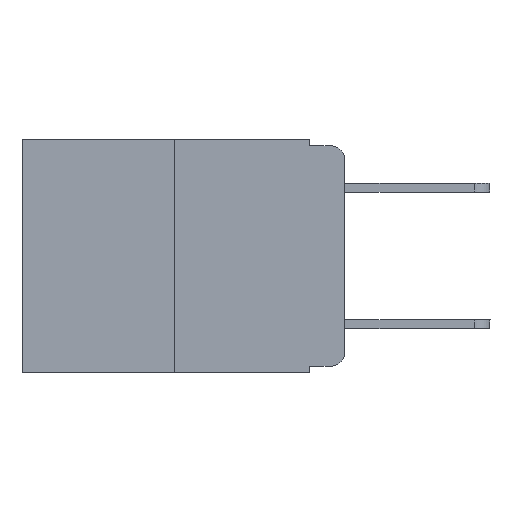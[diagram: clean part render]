
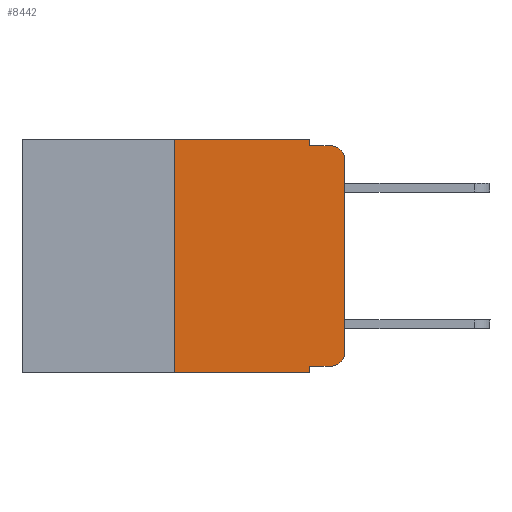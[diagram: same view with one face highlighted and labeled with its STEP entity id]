
A CAD part, left-side view. The second image highlights one B-rep face of the part: STEP entity #8442.
In plain terms, the highlighted planar face has unit normal (-1, 0, 0).
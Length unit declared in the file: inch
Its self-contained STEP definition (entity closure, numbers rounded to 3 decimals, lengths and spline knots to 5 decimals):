
#115 = LINE ( 'NONE', #10864, #8939 ) ;
#200 = LINE ( 'NONE', #6175, #12722 ) ;
#201 = EDGE_CURVE ( 'NONE', #2039, #1813, #435, .T. ) ;
#435 = LINE ( 'NONE', #6484, #12505 ) ;
#469 = ORIENTED_EDGE ( 'NONE', *, *, #7797, .T. ) ;
#483 = VECTOR ( 'NONE', #10882, 39.37008 ) ;
#596 = DIRECTION ( 'NONE',  ( 0., -1., 0. ) ) ;
#597 = CARTESIAN_POINT ( 'NONE',  ( 0., 0.051, -0.333 ) ) ;
#646 = DIRECTION ( 'NONE',  ( 0., -1., 0. ) ) ;
#672 = AXIS2_PLACEMENT_3D ( 'NONE', #8662, #4811, #8749 ) ;
#1133 = ORIENTED_EDGE ( 'NONE', *, *, #11712, .T. ) ;
#1342 = EDGE_LOOP ( 'NONE', ( #6219, #469, #8096, #11577, #10101, #4551, #4410, #12047, #10363, #1133 ) ) ;
#1742 = VECTOR ( 'NONE', #646, 39.37008 ) ;
#1813 = VERTEX_POINT ( 'NONE', #3310 ) ;
#1833 = CARTESIAN_POINT ( 'NONE',  ( 0., 0.25, -0.343 ) ) ;
#1901 = CARTESIAN_POINT ( 'NONE',  ( 0., 0.25, 0. ) ) ;
#1926 = VERTEX_POINT ( 'NONE', #1833 ) ;
#2039 = VERTEX_POINT ( 'NONE', #8715 ) ;
#2201 = VERTEX_POINT ( 'NONE', #11887 ) ;
#2207 = LINE ( 'NONE', #4011, #483 ) ;
#2269 = CARTESIAN_POINT ( 'NONE',  ( 0., 0., -0.03 ) ) ;
#2377 = CIRCLE ( 'NONE', #8976, 0.02 ) ;
#2406 = CARTESIAN_POINT ( 'NONE',  ( 0., 0., -0.313 ) ) ;
#2563 = LINE ( 'NONE', #6766, #8119 ) ;
#3084 = DIRECTION ( 'NONE',  ( 0., 0., 1. ) ) ;
#3139 = EDGE_CURVE ( 'NONE', #2201, #9923, #11011, .T. ) ;
#3310 = CARTESIAN_POINT ( 'NONE',  ( 0., 0.051, -0.01 ) ) ;
#3576 = VERTEX_POINT ( 'NONE', #2269 ) ;
#3888 = EDGE_CURVE ( 'NONE', #8419, #2039, #6986, .T. ) ;
#4011 = CARTESIAN_POINT ( 'NONE',  ( 0., 0.051, -0.01 ) ) ;
#4060 = LINE ( 'NONE', #8194, #5748 ) ;
#4410 = ORIENTED_EDGE ( 'NONE', *, *, #9126, .T. ) ;
#4491 = CIRCLE ( 'NONE', #672, 0.02 ) ;
#4504 = VERTEX_POINT ( 'NONE', #12550 ) ;
#4551 = ORIENTED_EDGE ( 'NONE', *, *, #7932, .F. ) ;
#4811 = DIRECTION ( 'NONE',  ( -1., 0., 0. ) ) ;
#5748 = VECTOR ( 'NONE', #9230, 39.37008 ) ;
#6021 = VERTEX_POINT ( 'NONE', #9377 ) ;
#6175 = CARTESIAN_POINT ( 'NONE',  ( 0., 0., 0. ) ) ;
#6219 = ORIENTED_EDGE ( 'NONE', *, *, #10910, .T. ) ;
#6456 = DIRECTION ( 'NONE',  ( -1., 0., 0. ) ) ;
#6484 = CARTESIAN_POINT ( 'NONE',  ( 0., 0.051, 0. ) ) ;
#6487 = CARTESIAN_POINT ( 'NONE',  ( 0., 0.02, -0.313 ) ) ;
#6766 = CARTESIAN_POINT ( 'NONE',  ( 0., 0.473, -0.343 ) ) ;
#6986 = LINE ( 'NONE', #10093, #1742 ) ;
#7739 = DIRECTION ( 'NONE',  ( 0., 0., -1. ) ) ;
#7797 = EDGE_CURVE ( 'NONE', #3576, #4504, #4491, .T. ) ;
#7932 = EDGE_CURVE ( 'NONE', #1926, #8419, #115, .T. ) ;
#8096 = ORIENTED_EDGE ( 'NONE', *, *, #11501, .F. ) ;
#8119 = VECTOR ( 'NONE', #596, 39.37008 ) ;
#8194 = CARTESIAN_POINT ( 'NONE',  ( 0., 0.051, 0. ) ) ;
#8419 = VERTEX_POINT ( 'NONE', #1901 ) ;
#8442 = ADVANCED_FACE ( 'NONE', ( #9376 ), #8820, .F. ) ;
#8536 = DIRECTION ( 'NONE',  ( 0., 0., -1. ) ) ;
#8662 = CARTESIAN_POINT ( 'NONE',  ( 0., 0.02, -0.03 ) ) ;
#8715 = CARTESIAN_POINT ( 'NONE',  ( 0., 0.051, 0. ) ) ;
#8739 = DIRECTION ( 'NONE',  ( 1., 0., 0. ) ) ;
#8749 = DIRECTION ( 'NONE',  ( 0., 0., -1. ) ) ;
#8820 = PLANE ( 'NONE',  #11857 ) ;
#8939 = VECTOR ( 'NONE', #3084, 39.37008 ) ;
#8976 = AXIS2_PLACEMENT_3D ( 'NONE', #6487, #6456, #10394 ) ;
#9126 = EDGE_CURVE ( 'NONE', #1926, #6021, #2563, .T. ) ;
#9230 = DIRECTION ( 'NONE',  ( 0., 0., -1. ) ) ;
#9376 = FACE_OUTER_BOUND ( 'NONE', #1342, .T. ) ;
#9377 = CARTESIAN_POINT ( 'NONE',  ( 0., 0.051, -0.343 ) ) ;
#9764 = VECTOR ( 'NONE', #10565, 39.37008 ) ;
#9923 = VERTEX_POINT ( 'NONE', #10832 ) ;
#9950 = DIRECTION ( 'NONE',  ( 0., 0., 1. ) ) ;
#10093 = CARTESIAN_POINT ( 'NONE',  ( 0., 0.473, 0. ) ) ;
#10101 = ORIENTED_EDGE ( 'NONE', *, *, #3888, .F. ) ;
#10284 = VERTEX_POINT ( 'NONE', #2406 ) ;
#10363 = ORIENTED_EDGE ( 'NONE', *, *, #3139, .T. ) ;
#10394 = DIRECTION ( 'NONE',  ( 0., 0., -1. ) ) ;
#10565 = DIRECTION ( 'NONE',  ( 0., -1., 0. ) ) ;
#10832 = CARTESIAN_POINT ( 'NONE',  ( 0., 0.02, -0.333 ) ) ;
#10864 = CARTESIAN_POINT ( 'NONE',  ( 0., 0.25, 0. ) ) ;
#10882 = DIRECTION ( 'NONE',  ( 0., -1., 0. ) ) ;
#10910 = EDGE_CURVE ( 'NONE', #10284, #3576, #200, .T. ) ;
#11011 = LINE ( 'NONE', #597, #9764 ) ;
#11501 = EDGE_CURVE ( 'NONE', #1813, #4504, #2207, .T. ) ;
#11577 = ORIENTED_EDGE ( 'NONE', *, *, #201, .F. ) ;
#11679 = CARTESIAN_POINT ( 'NONE',  ( 0., 0.473, 0. ) ) ;
#11712 = EDGE_CURVE ( 'NONE', #9923, #10284, #2377, .T. ) ;
#11857 = AXIS2_PLACEMENT_3D ( 'NONE', #11679, #8739, #7739 ) ;
#11887 = CARTESIAN_POINT ( 'NONE',  ( 0., 0.051, -0.333 ) ) ;
#12047 = ORIENTED_EDGE ( 'NONE', *, *, #12521, .F. ) ;
#12505 = VECTOR ( 'NONE', #8536, 39.37008 ) ;
#12521 = EDGE_CURVE ( 'NONE', #2201, #6021, #4060, .T. ) ;
#12550 = CARTESIAN_POINT ( 'NONE',  ( 0., 0.02, -0.01 ) ) ;
#12722 = VECTOR ( 'NONE', #9950, 39.37008 ) ;
